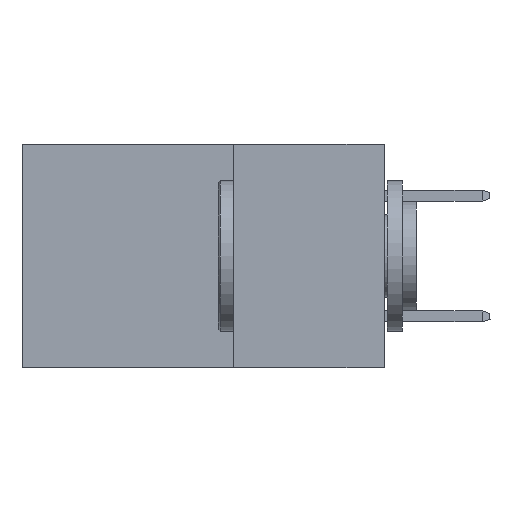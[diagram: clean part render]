
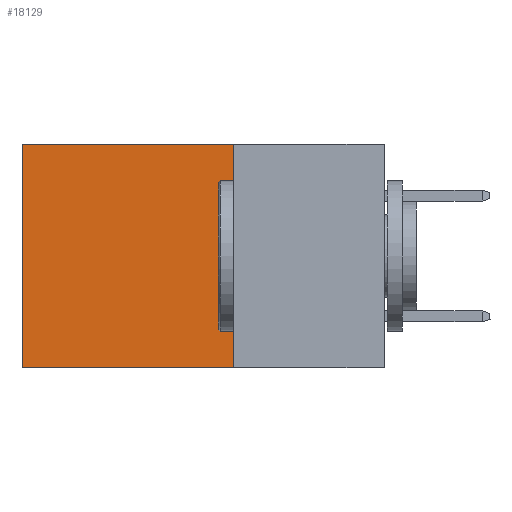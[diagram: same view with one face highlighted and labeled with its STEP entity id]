
A CAD part, left-side view. The second image highlights one B-rep face of the part: STEP entity #18129.
In plain terms, the highlighted planar face has unit normal (-1, 0, 0).
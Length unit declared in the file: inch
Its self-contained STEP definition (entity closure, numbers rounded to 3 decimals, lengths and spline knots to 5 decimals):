
#417 = VECTOR ( 'NONE', #18597, 39.37008 ) ;
#1003 = LINE ( 'NONE', #7358, #417 ) ;
#1631 = EDGE_CURVE ( 'NONE', #18438, #19648, #22118, .T. ) ;
#1804 = DIRECTION ( 'NONE',  ( 0., 0., -1. ) ) ;
#2763 = VECTOR ( 'NONE', #17212, 39.37008 ) ;
#2985 = CARTESIAN_POINT ( 'NONE',  ( 0.2615, 0.25, -0.37 ) ) ;
#3894 = EDGE_CURVE ( 'NONE', #7857, #5704, #6802, .T. ) ;
#4860 = DIRECTION ( 'NONE',  ( 0., 0., -1. ) ) ;
#5476 = CARTESIAN_POINT ( 'NONE',  ( 0.2615, 0.6, -0.37 ) ) ;
#5704 = VERTEX_POINT ( 'NONE', #13035 ) ;
#6802 = LINE ( 'NONE', #19592, #21175 ) ;
#6936 = ORIENTED_EDGE ( 'NONE', *, *, #18356, .F. ) ;
#7358 = CARTESIAN_POINT ( 'NONE',  ( 0.2615, 0.25, -0.37 ) ) ;
#7624 = AXIS2_PLACEMENT_3D ( 'NONE', #2985, #16168, #4860 ) ;
#7857 = VERTEX_POINT ( 'NONE', #13519 ) ;
#9293 = VECTOR ( 'NONE', #1804, 39.37008 ) ;
#12376 = PLANE ( 'NONE',  #7624 ) ;
#13035 = CARTESIAN_POINT ( 'NONE',  ( 0.2615, 0.6, -0.37 ) ) ;
#13519 = CARTESIAN_POINT ( 'NONE',  ( 0.2615, 0.25, -0.37 ) ) ;
#14421 = CARTESIAN_POINT ( 'NONE',  ( 0.2615, 0.25, 0. ) ) ;
#15080 = CARTESIAN_POINT ( 'NONE',  ( 0.2615, 0.25, 0. ) ) ;
#16168 = DIRECTION ( 'NONE',  ( 1., 0., 0. ) ) ;
#17212 = DIRECTION ( 'NONE',  ( 0., 1., 0. ) ) ;
#18129 = ADVANCED_FACE ( 'NONE', ( #20095 ), #12376, .F. ) ;
#18356 = EDGE_CURVE ( 'NONE', #18438, #7857, #1003, .T. ) ;
#18438 = VERTEX_POINT ( 'NONE', #15080 ) ;
#18597 = DIRECTION ( 'NONE',  ( 0., 0., -1. ) ) ;
#19099 = DIRECTION ( 'NONE',  ( 0., 1., 0. ) ) ;
#19160 = ORIENTED_EDGE ( 'NONE', *, *, #1631, .T. ) ;
#19592 = CARTESIAN_POINT ( 'NONE',  ( 0.2615, 0.25, -0.37 ) ) ;
#19648 = VERTEX_POINT ( 'NONE', #20260 ) ;
#19789 = ORIENTED_EDGE ( 'NONE', *, *, #3894, .F. ) ;
#20095 = FACE_OUTER_BOUND ( 'NONE', #22645, .T. ) ;
#20260 = CARTESIAN_POINT ( 'NONE',  ( 0.2615, 0.6, 0. ) ) ;
#21175 = VECTOR ( 'NONE', #19099, 39.37008 ) ;
#22118 = LINE ( 'NONE', #14421, #2763 ) ;
#22645 = EDGE_LOOP ( 'NONE', ( #23111, #19789, #6936, #19160 ) ) ;
#23111 = ORIENTED_EDGE ( 'NONE', *, *, #23628, .T. ) ;
#23558 = LINE ( 'NONE', #5476, #9293 ) ;
#23628 = EDGE_CURVE ( 'NONE', #19648, #5704, #23558, .T. ) ;
